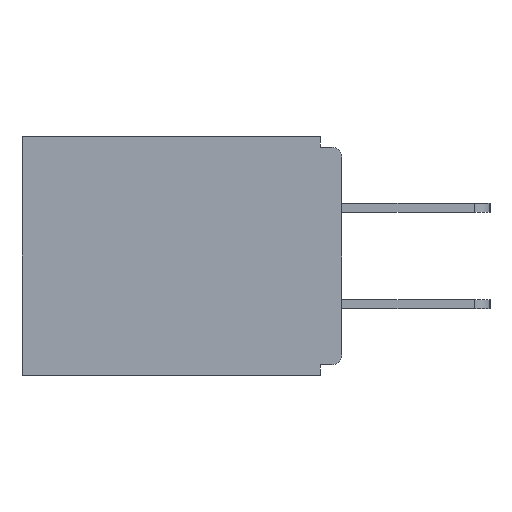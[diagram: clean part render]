
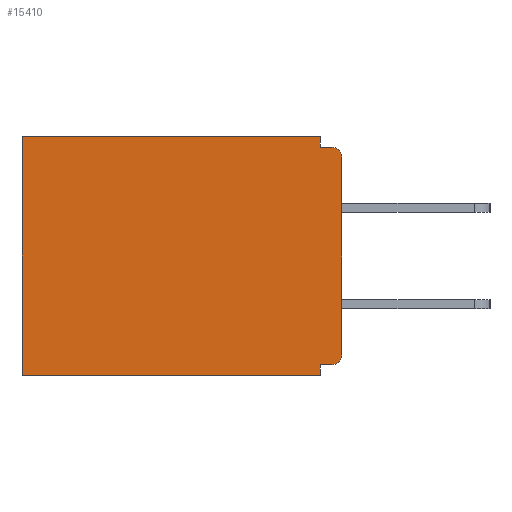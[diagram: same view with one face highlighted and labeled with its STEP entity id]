
A CAD part, left-side view. The second image highlights one B-rep face of the part: STEP entity #15410.
In plain terms, the highlighted planar face has unit normal (-1, 0, 0).
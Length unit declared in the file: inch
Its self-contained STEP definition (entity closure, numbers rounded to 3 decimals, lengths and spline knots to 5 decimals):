
#250 = VERTEX_POINT ( 'NONE', #3160 ) ;
#533 = EDGE_CURVE ( 'NONE', #15386, #8589, #15780, .T. ) ;
#877 = DIRECTION ( 'NONE',  ( 0., 0., -1. ) ) ;
#1153 = EDGE_CURVE ( 'NONE', #14263, #5661, #20837, .T. ) ;
#1178 = CARTESIAN_POINT ( 'NONE',  ( 0.298, 0.015, -0.313 ) ) ;
#1321 = ORIENTED_EDGE ( 'NONE', *, *, #533, .F. ) ;
#1693 = ORIENTED_EDGE ( 'NONE', *, *, #5835, .F. ) ;
#2532 = DIRECTION ( 'NONE',  ( -1., 0., 0. ) ) ;
#2943 = CARTESIAN_POINT ( 'NONE',  ( 0.298, 0., 0. ) ) ;
#3160 = CARTESIAN_POINT ( 'NONE',  ( 0.298, 0.46, 0. ) ) ;
#3165 = DIRECTION ( 'NONE',  ( 0., 1., 0. ) ) ;
#3229 = DIRECTION ( 'NONE',  ( 0., -1., 0. ) ) ;
#4299 = CARTESIAN_POINT ( 'NONE',  ( 0.298, 0.031, -0.343 ) ) ;
#4358 = CARTESIAN_POINT ( 'NONE',  ( 0.298, 0.015, -0.328 ) ) ;
#4428 = CARTESIAN_POINT ( 'NONE',  ( 0.298, 0.031, -0.015 ) ) ;
#4591 = AXIS2_PLACEMENT_3D ( 'NONE', #2943, #8056, #21760 ) ;
#4825 = DIRECTION ( 'NONE',  ( 0., 0., -1. ) ) ;
#4846 = ORIENTED_EDGE ( 'NONE', *, *, #1153, .F. ) ;
#4848 = LINE ( 'NONE', #13688, #14962 ) ;
#5013 = ORIENTED_EDGE ( 'NONE', *, *, #17647, .T. ) ;
#5124 = EDGE_CURVE ( 'NONE', #18439, #250, #8156, .T. ) ;
#5133 = CARTESIAN_POINT ( 'NONE',  ( 0.298, 0.031, 0. ) ) ;
#5215 = VECTOR ( 'NONE', #3165, 39.37008 ) ;
#5447 = LINE ( 'NONE', #10943, #9138 ) ;
#5585 = CARTESIAN_POINT ( 'NONE',  ( 0.298, 0., -0.328 ) ) ;
#5621 = DIRECTION ( 'NONE',  ( 0., 0., -1. ) ) ;
#5661 = VERTEX_POINT ( 'NONE', #6017 ) ;
#5750 = CARTESIAN_POINT ( 'NONE',  ( 0.298, 0.015, -0.03 ) ) ;
#5835 = EDGE_CURVE ( 'NONE', #18439, #15386, #5447, .T. ) ;
#6017 = CARTESIAN_POINT ( 'NONE',  ( 0.298, 0.46, -0.343 ) ) ;
#6161 = LINE ( 'NONE', #5585, #18943 ) ;
#6665 = VECTOR ( 'NONE', #11077, 39.37008 ) ;
#6688 = CARTESIAN_POINT ( 'NONE',  ( 0.298, 0., 0. ) ) ;
#7045 = DIRECTION ( 'NONE',  ( 0., 1., 0. ) ) ;
#7460 = ORIENTED_EDGE ( 'NONE', *, *, #16213, .T. ) ;
#7500 = VECTOR ( 'NONE', #7045, 39.37008 ) ;
#7720 = CARTESIAN_POINT ( 'NONE',  ( 0.298, 0.015, -0.015 ) ) ;
#7835 = VERTEX_POINT ( 'NONE', #4358 ) ;
#8056 = DIRECTION ( 'NONE',  ( 1., 0., 0. ) ) ;
#8082 = VECTOR ( 'NONE', #3229, 39.37008 ) ;
#8116 = CIRCLE ( 'NONE', #8256, 0.015 ) ;
#8156 = LINE ( 'NONE', #18582, #5215 ) ;
#8256 = AXIS2_PLACEMENT_3D ( 'NONE', #5750, #16109, #12757 ) ;
#8338 = VERTEX_POINT ( 'NONE', #15080 ) ;
#8397 = VERTEX_POINT ( 'NONE', #13454 ) ;
#8589 = VERTEX_POINT ( 'NONE', #7720 ) ;
#8632 = ORIENTED_EDGE ( 'NONE', *, *, #10982, .F. ) ;
#9138 = VECTOR ( 'NONE', #5621, 39.37008 ) ;
#9657 = CARTESIAN_POINT ( 'NONE',  ( 0.298, 0.031, -0.343 ) ) ;
#9880 = PLANE ( 'NONE',  #4591 ) ;
#9995 = ORIENTED_EDGE ( 'NONE', *, *, #17640, .F. ) ;
#10438 = DIRECTION ( 'NONE',  ( 0., 0., -1. ) ) ;
#10943 = CARTESIAN_POINT ( 'NONE',  ( 0.298, 0.031, -0.343 ) ) ;
#10982 = EDGE_CURVE ( 'NONE', #7835, #18097, #6161, .T. ) ;
#11077 = DIRECTION ( 'NONE',  ( 0., 0., -1. ) ) ;
#11214 = LINE ( 'NONE', #9657, #6665 ) ;
#12757 = DIRECTION ( 'NONE',  ( 0., 0., -1. ) ) ;
#12979 = EDGE_CURVE ( 'NONE', #8338, #8397, #18845, .T. ) ;
#13003 = VECTOR ( 'NONE', #4825, 39.37008 ) ;
#13301 = ORIENTED_EDGE ( 'NONE', *, *, #12979, .F. ) ;
#13454 = CARTESIAN_POINT ( 'NONE',  ( 0.298, 0., -0.313 ) ) ;
#13688 = CARTESIAN_POINT ( 'NONE',  ( 0.298, 0.46, 0. ) ) ;
#14263 = VERTEX_POINT ( 'NONE', #4299 ) ;
#14874 = CARTESIAN_POINT ( 'NONE',  ( 0.298, 0., -0.015 ) ) ;
#14962 = VECTOR ( 'NONE', #10438, 39.37008 ) ;
#15080 = CARTESIAN_POINT ( 'NONE',  ( 0.298, 0., -0.03 ) ) ;
#15386 = VERTEX_POINT ( 'NONE', #4428 ) ;
#15410 = ADVANCED_FACE ( 'NONE', ( #15794 ), #9880, .F. ) ;
#15434 = CARTESIAN_POINT ( 'NONE',  ( 0.298, 0., -0.343 ) ) ;
#15577 = EDGE_LOOP ( 'NONE', ( #18660, #1321, #1693, #18293, #7460, #4846, #9995, #8632, #5013, #13301 ) ) ;
#15641 = DIRECTION ( 'NONE',  ( 0., 1., 0. ) ) ;
#15780 = LINE ( 'NONE', #14874, #8082 ) ;
#15794 = FACE_OUTER_BOUND ( 'NONE', #15577, .T. ) ;
#16109 = DIRECTION ( 'NONE',  ( -1., 0., 0. ) ) ;
#16213 = EDGE_CURVE ( 'NONE', #250, #5661, #4848, .T. ) ;
#17640 = EDGE_CURVE ( 'NONE', #18097, #14263, #11214, .T. ) ;
#17647 = EDGE_CURVE ( 'NONE', #7835, #8397, #21315, .T. ) ;
#18097 = VERTEX_POINT ( 'NONE', #20207 ) ;
#18293 = ORIENTED_EDGE ( 'NONE', *, *, #5124, .T. ) ;
#18439 = VERTEX_POINT ( 'NONE', #5133 ) ;
#18582 = CARTESIAN_POINT ( 'NONE',  ( 0.298, 0., 0. ) ) ;
#18660 = ORIENTED_EDGE ( 'NONE', *, *, #21954, .T. ) ;
#18717 = AXIS2_PLACEMENT_3D ( 'NONE', #1178, #2532, #877 ) ;
#18845 = LINE ( 'NONE', #6688, #13003 ) ;
#18943 = VECTOR ( 'NONE', #15641, 39.37008 ) ;
#20207 = CARTESIAN_POINT ( 'NONE',  ( 0.298, 0.031, -0.328 ) ) ;
#20837 = LINE ( 'NONE', #15434, #7500 ) ;
#21315 = CIRCLE ( 'NONE', #18717, 0.015 ) ;
#21760 = DIRECTION ( 'NONE',  ( 0., 0., -1. ) ) ;
#21954 = EDGE_CURVE ( 'NONE', #8338, #8589, #8116, .T. ) ;
